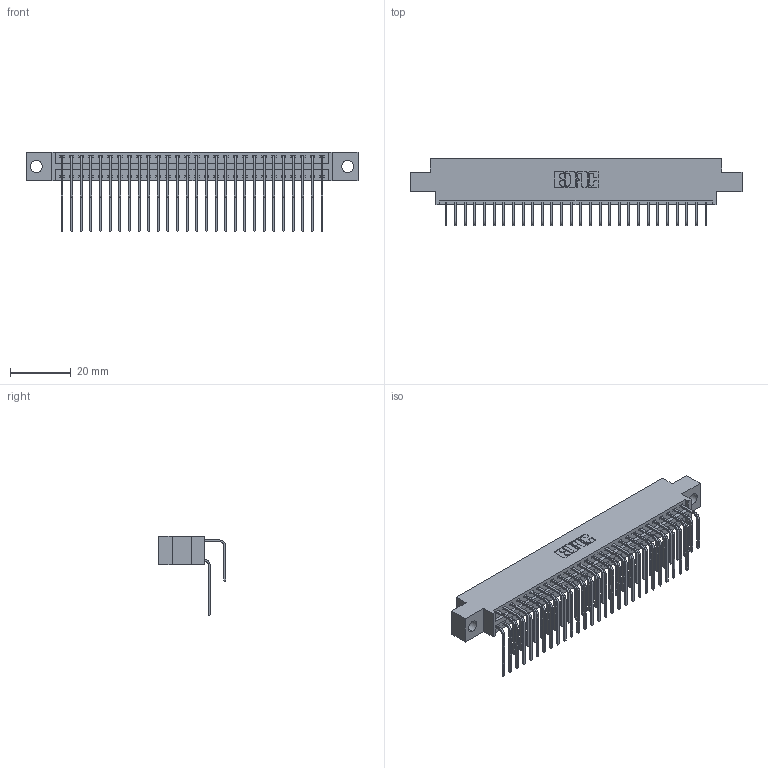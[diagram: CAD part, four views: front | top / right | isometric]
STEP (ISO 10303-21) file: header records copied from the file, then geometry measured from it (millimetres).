
FILE_DESCRIPTION (( 'STEP AP203' ), '1' );
FILE_NAME ('396-056-558-804.STEP', '2018-09-08T10:23:17', ( '' ), ( '' ), 'SwSTEP 2.0', 'SolidWorks 2016', '' );
FILE_SCHEMA (( 'CONFIG_CONTROL_DESIGN' ));
Length unit declared in the file: inch
Products named in the file (4): 396-056-558-804; 346 Part_0.170 Offset - 0.156 Dia-TH; 345-292-001_558 559 Tail - 1; 345-292-001_558 Tail - 2
Assembly tree (57 placements, depth 2):
  396-056-558-804
    346 Part_0.170 Offset - 0.156 Dia-TH
    345-292-001_558 559 Tail - 1  x28
    345-292-001_558 Tail - 2  x28
Bounding box: 109.47 x 22.16 x 26.16 mm (x, y, z)
Volume: 10646.9 mm3; surface area: 15957.6 mm2
Topology: 57 solids, 57 shells, 3150 faces, 9357 edges, 6162 vertices
Faces by surface type: plane 2152, cylinder 998
Entity records: 22077 total; most frequent: CARTESIAN_POINT 3711, ORIENTED_EDGE 3594, DIRECTION 3293, EDGE_CURVE 1797, LINE 1513, VECTOR 1513, VERTEX_POINT 1194, AXIS2_PLACEMENT_3D 890
